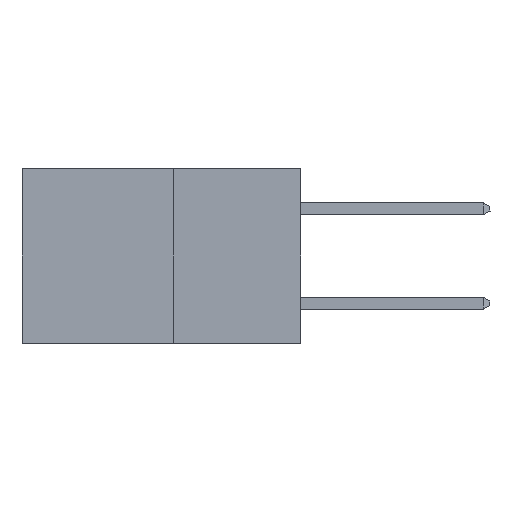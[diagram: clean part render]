
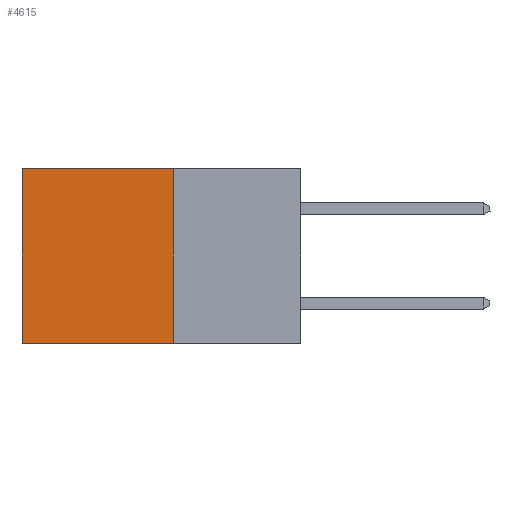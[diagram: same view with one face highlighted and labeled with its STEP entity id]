
A CAD part, left-side view. The second image highlights one B-rep face of the part: STEP entity #4615.
In plain terms, the highlighted planar face has unit normal (-1, 0, 0).
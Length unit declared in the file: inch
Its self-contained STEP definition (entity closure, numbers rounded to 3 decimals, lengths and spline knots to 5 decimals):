
#1325 = VECTOR ( 'NONE', #1873, 39.37008 ) ;
#1386 = CARTESIAN_POINT ( 'NONE',  ( 0.277, 0.27, 0. ) ) ;
#1606 = ORIENTED_EDGE ( 'NONE', *, *, #9036, .F. ) ;
#1643 = DIRECTION ( 'NONE',  ( 0., 1., 0. ) ) ;
#1860 = ORIENTED_EDGE ( 'NONE', *, *, #5433, .F. ) ;
#1873 = DIRECTION ( 'NONE',  ( 0., 0., -1. ) ) ;
#3298 = VERTEX_POINT ( 'NONE', #1386 ) ;
#4007 = VECTOR ( 'NONE', #11768, 39.37008 ) ;
#4094 = VECTOR ( 'NONE', #1643, 39.37008 ) ;
#4615 = ADVANCED_FACE ( 'NONE', ( #6015 ), #17891, .F. ) ;
#5433 = EDGE_CURVE ( 'NONE', #17353, #15324, #7941, .T. ) ;
#5630 = CARTESIAN_POINT ( 'NONE',  ( 0.277, 0.59, -0.37 ) ) ;
#6015 = FACE_OUTER_BOUND ( 'NONE', #13227, .T. ) ;
#6978 = VECTOR ( 'NONE', #17497, 39.37008 ) ;
#7509 = CARTESIAN_POINT ( 'NONE',  ( 0.277, 0.27, -0.37 ) ) ;
#7512 = CARTESIAN_POINT ( 'NONE',  ( 0.277, 0.27, -0.37 ) ) ;
#7597 = EDGE_CURVE ( 'NONE', #3298, #11012, #15596, .T. ) ;
#7855 = DIRECTION ( 'NONE',  ( 0., 0., -1. ) ) ;
#7941 = LINE ( 'NONE', #8551, #4094 ) ;
#8551 = CARTESIAN_POINT ( 'NONE',  ( 0.277, 0.27, -0.37 ) ) ;
#8723 = AXIS2_PLACEMENT_3D ( 'NONE', #7509, #14940, #7855 ) ;
#8776 = CARTESIAN_POINT ( 'NONE',  ( 0.277, 0.59, -0.37 ) ) ;
#9036 = EDGE_CURVE ( 'NONE', #3298, #17353, #12804, .T. ) ;
#9686 = CARTESIAN_POINT ( 'NONE',  ( 0.277, 0.27, 0. ) ) ;
#10355 = ORIENTED_EDGE ( 'NONE', *, *, #15449, .T. ) ;
#11012 = VERTEX_POINT ( 'NONE', #18194 ) ;
#11296 = LINE ( 'NONE', #8776, #6978 ) ;
#11768 = DIRECTION ( 'NONE',  ( 0., 1., 0. ) ) ;
#12422 = CARTESIAN_POINT ( 'NONE',  ( 0.277, 0.27, -0.37 ) ) ;
#12804 = LINE ( 'NONE', #7512, #1325 ) ;
#13227 = EDGE_LOOP ( 'NONE', ( #10355, #1860, #1606, #16834 ) ) ;
#14940 = DIRECTION ( 'NONE',  ( 1., 0., 0. ) ) ;
#15324 = VERTEX_POINT ( 'NONE', #5630 ) ;
#15449 = EDGE_CURVE ( 'NONE', #11012, #15324, #11296, .T. ) ;
#15596 = LINE ( 'NONE', #9686, #4007 ) ;
#16834 = ORIENTED_EDGE ( 'NONE', *, *, #7597, .T. ) ;
#17353 = VERTEX_POINT ( 'NONE', #12422 ) ;
#17497 = DIRECTION ( 'NONE',  ( 0., 0., -1. ) ) ;
#17891 = PLANE ( 'NONE',  #8723 ) ;
#18194 = CARTESIAN_POINT ( 'NONE',  ( 0.277, 0.59, 0. ) ) ;
